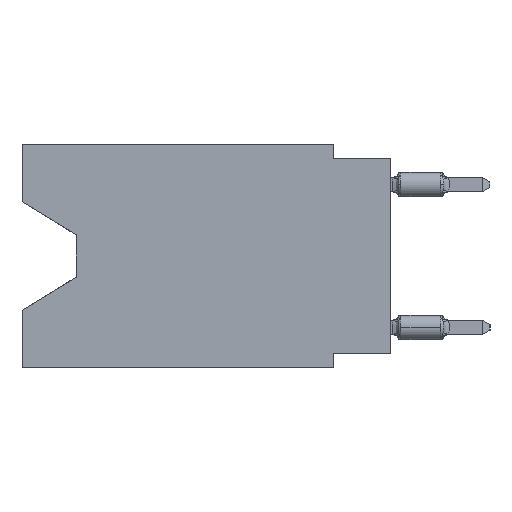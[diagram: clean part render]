
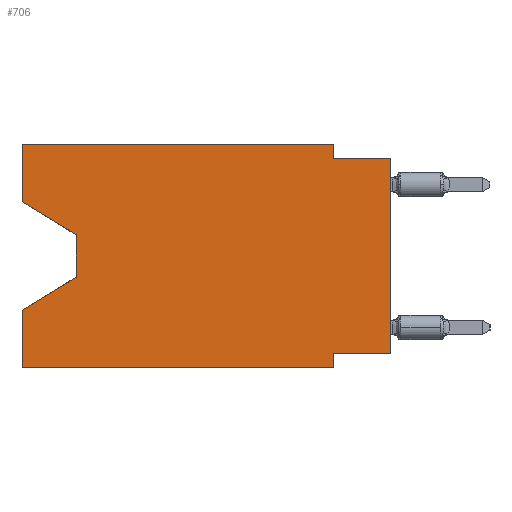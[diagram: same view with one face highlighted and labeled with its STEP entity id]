
A CAD part, left-side view. The second image highlights one B-rep face of the part: STEP entity #706.
In plain terms, the highlighted planar face has unit normal (-1, 0, 0).
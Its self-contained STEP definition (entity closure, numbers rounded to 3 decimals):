
#27 = ORIENTED_EDGE ( 'NONE', *, *, #21174, .T. ) ;
#43 = ORIENTED_EDGE ( 'NONE', *, *, #28052, .F. ) ;
#706 = ADVANCED_FACE ( 'NONE', ( #11646 ), #8113, .F. ) ;
#1890 = DIRECTION ( 'NONE',  ( 0., 0., -1. ) ) ;
#2440 = ORIENTED_EDGE ( 'NONE', *, *, #31169, .F. ) ;
#2539 = VECTOR ( 'NONE', #29203, 1000. ) ;
#2676 = VECTOR ( 'NONE', #26669, 1000. ) ;
#3060 = DIRECTION ( 'NONE',  ( 0., -1., 0. ) ) ;
#3072 = CARTESIAN_POINT ( 'NONE',  ( 0., 0., -0.635 ) ) ;
#3345 = ORIENTED_EDGE ( 'NONE', *, *, #27462, .T. ) ;
#3545 = VERTEX_POINT ( 'NONE', #33434 ) ;
#3984 = CARTESIAN_POINT ( 'NONE',  ( 0., 2.54, 0. ) ) ;
#4119 = AXIS2_PLACEMENT_3D ( 'NONE', #33405, #30606, #16487 ) ;
#4526 = CARTESIAN_POINT ( 'NONE',  ( 0., 13.97, -4.013 ) ) ;
#5531 = CARTESIAN_POINT ( 'NONE',  ( 0., 16.383, -2.546 ) ) ;
#6241 = DIRECTION ( 'NONE',  ( 0., -1., 0. ) ) ;
#6780 = CARTESIAN_POINT ( 'NONE',  ( 0., 16.383, 0. ) ) ;
#6974 = DIRECTION ( 'NONE',  ( 0., 0., 1. ) ) ;
#6982 = DIRECTION ( 'NONE',  ( 0., 0., 1. ) ) ;
#7570 = VERTEX_POINT ( 'NONE', #23648 ) ;
#8062 = CARTESIAN_POINT ( 'NONE',  ( 0., 13.97, -5.893 ) ) ;
#8113 = PLANE ( 'NONE',  #4119 ) ;
#8251 = LINE ( 'NONE', #33184, #9685 ) ;
#8292 = VERTEX_POINT ( 'NONE', #19841 ) ;
#8671 = EDGE_CURVE ( 'NONE', #15318, #7570, #36759, .T. ) ;
#9033 = LINE ( 'NONE', #29667, #34052 ) ;
#9123 = CARTESIAN_POINT ( 'NONE',  ( 0., 2.54, -9.906 ) ) ;
#9231 = CARTESIAN_POINT ( 'NONE',  ( 0., 0., -9.271 ) ) ;
#9255 = CARTESIAN_POINT ( 'NONE',  ( 0., 16.383, 0. ) ) ;
#9277 = VECTOR ( 'NONE', #35821, 1000. ) ;
#9545 = CARTESIAN_POINT ( 'NONE',  ( 0., 16.383, 0. ) ) ;
#9685 = VECTOR ( 'NONE', #27785, 1000. ) ;
#10283 = LINE ( 'NONE', #4526, #21784 ) ;
#10289 = DIRECTION ( 'NONE',  ( 0., 0., 1. ) ) ;
#11170 = VERTEX_POINT ( 'NONE', #9255 ) ;
#11646 = FACE_OUTER_BOUND ( 'NONE', #32941, .T. ) ;
#12085 = VERTEX_POINT ( 'NONE', #32908 ) ;
#14298 = ORIENTED_EDGE ( 'NONE', *, *, #34513, .T. ) ;
#14476 = LINE ( 'NONE', #31404, #17325 ) ;
#14678 = DIRECTION ( 'NONE',  ( 0., 0.855, -0.519 ) ) ;
#14992 = VERTEX_POINT ( 'NONE', #8062 ) ;
#15318 = VERTEX_POINT ( 'NONE', #5531 ) ;
#15485 = CARTESIAN_POINT ( 'NONE',  ( 0., 2.54, -9.271 ) ) ;
#15850 = CARTESIAN_POINT ( 'NONE',  ( 0., 0., -0.635 ) ) ;
#16077 = ORIENTED_EDGE ( 'NONE', *, *, #29235, .F. ) ;
#16335 = VECTOR ( 'NONE', #6241, 1000. ) ;
#16487 = DIRECTION ( 'NONE',  ( 0., 0., -1. ) ) ;
#17028 = ORIENTED_EDGE ( 'NONE', *, *, #23707, .T. ) ;
#17325 = VECTOR ( 'NONE', #14678, 1000. ) ;
#17395 = LINE ( 'NONE', #23345, #28670 ) ;
#18206 = VERTEX_POINT ( 'NONE', #3984 ) ;
#18672 = LINE ( 'NONE', #24428, #32386 ) ;
#19533 = VERTEX_POINT ( 'NONE', #9231 ) ;
#19618 = CARTESIAN_POINT ( 'NONE',  ( 0., 16.383, -2.546 ) ) ;
#19841 = CARTESIAN_POINT ( 'NONE',  ( 0., 2.54, -9.906 ) ) ;
#21174 = EDGE_CURVE ( 'NONE', #7570, #14992, #10283, .T. ) ;
#21487 = ORIENTED_EDGE ( 'NONE', *, *, #32531, .F. ) ;
#21784 = VECTOR ( 'NONE', #1890, 1000. ) ;
#22774 = ORIENTED_EDGE ( 'NONE', *, *, #8671, .T. ) ;
#23345 = CARTESIAN_POINT ( 'NONE',  ( 0., 16.383, -9.906 ) ) ;
#23648 = CARTESIAN_POINT ( 'NONE',  ( 0., 13.97, -4.013 ) ) ;
#23707 = EDGE_CURVE ( 'NONE', #3545, #8292, #17395, .T. ) ;
#23981 = EDGE_CURVE ( 'NONE', #19533, #28472, #8251, .T. ) ;
#24428 = CARTESIAN_POINT ( 'NONE',  ( 0., 0., 0. ) ) ;
#24539 = CARTESIAN_POINT ( 'NONE',  ( 0., 2.54, -0.635 ) ) ;
#25989 = LINE ( 'NONE', #3072, #16335 ) ;
#26669 = DIRECTION ( 'NONE',  ( 0., -1., 0. ) ) ;
#26869 = LINE ( 'NONE', #6780, #29229 ) ;
#26954 = ORIENTED_EDGE ( 'NONE', *, *, #33015, .F. ) ;
#27071 = CARTESIAN_POINT ( 'NONE',  ( 0., 2.54, 0. ) ) ;
#27259 = LINE ( 'NONE', #27071, #9277 ) ;
#27462 = EDGE_CURVE ( 'NONE', #14992, #12085, #14476, .T. ) ;
#27785 = DIRECTION ( 'NONE',  ( 0., 1., 0. ) ) ;
#28052 = EDGE_CURVE ( 'NONE', #3545, #12085, #26869, .T. ) ;
#28472 = VERTEX_POINT ( 'NONE', #15485 ) ;
#28670 = VECTOR ( 'NONE', #3060, 1000. ) ;
#28844 = EDGE_CURVE ( 'NONE', #28472, #8292, #34622, .T. ) ;
#29014 = VERTEX_POINT ( 'NONE', #24539 ) ;
#29203 = DIRECTION ( 'NONE',  ( 0., 0., -1. ) ) ;
#29229 = VECTOR ( 'NONE', #6974, 1000. ) ;
#29235 = EDGE_CURVE ( 'NONE', #15318, #11170, #9033, .T. ) ;
#29667 = CARTESIAN_POINT ( 'NONE',  ( 0., 16.383, 0. ) ) ;
#29917 = ORIENTED_EDGE ( 'NONE', *, *, #28844, .F. ) ;
#30221 = ORIENTED_EDGE ( 'NONE', *, *, #23981, .F. ) ;
#30579 = DIRECTION ( 'NONE',  ( 0., -0.855, -0.519 ) ) ;
#30606 = DIRECTION ( 'NONE',  ( 1., 0., 0. ) ) ;
#31169 = EDGE_CURVE ( 'NONE', #29014, #34903, #25989, .T. ) ;
#31404 = CARTESIAN_POINT ( 'NONE',  ( 0., 13.97, -5.893 ) ) ;
#32386 = VECTOR ( 'NONE', #10289, 1000. ) ;
#32531 = EDGE_CURVE ( 'NONE', #18206, #29014, #27259, .T. ) ;
#32908 = CARTESIAN_POINT ( 'NONE',  ( 0., 16.383, -7.36 ) ) ;
#32941 = EDGE_LOOP ( 'NONE', ( #22774, #27, #3345, #43, #17028, #29917, #30221, #14298, #2440, #21487, #26954, #16077 ) ) ;
#33015 = EDGE_CURVE ( 'NONE', #11170, #18206, #35043, .T. ) ;
#33184 = CARTESIAN_POINT ( 'NONE',  ( 0., 0., -9.271 ) ) ;
#33405 = CARTESIAN_POINT ( 'NONE',  ( 0., 16.383, 0. ) ) ;
#33434 = CARTESIAN_POINT ( 'NONE',  ( 0., 16.383, -9.906 ) ) ;
#33577 = VECTOR ( 'NONE', #30579, 1000. ) ;
#34052 = VECTOR ( 'NONE', #6982, 1000. ) ;
#34513 = EDGE_CURVE ( 'NONE', #19533, #34903, #18672, .T. ) ;
#34622 = LINE ( 'NONE', #9123, #2539 ) ;
#34903 = VERTEX_POINT ( 'NONE', #15850 ) ;
#35043 = LINE ( 'NONE', #9545, #2676 ) ;
#35821 = DIRECTION ( 'NONE',  ( 0., 0., -1. ) ) ;
#36759 = LINE ( 'NONE', #19618, #33577 ) ;
